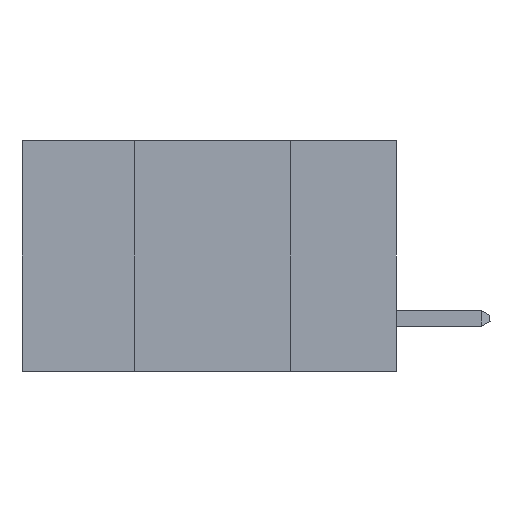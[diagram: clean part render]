
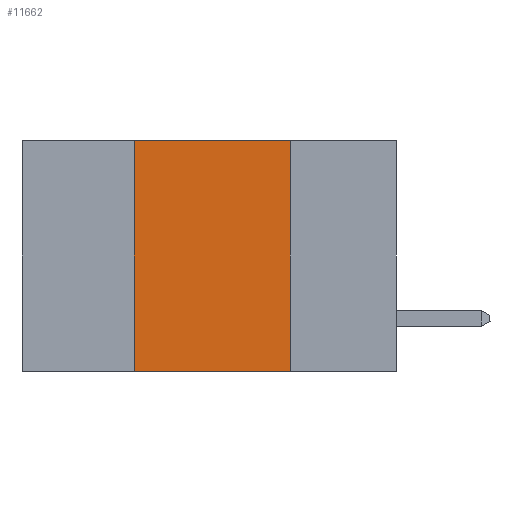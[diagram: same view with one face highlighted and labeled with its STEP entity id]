
A CAD part, left-side view. The second image highlights one B-rep face of the part: STEP entity #11662.
In plain terms, the highlighted planar face has unit normal (-1, 0, 0).
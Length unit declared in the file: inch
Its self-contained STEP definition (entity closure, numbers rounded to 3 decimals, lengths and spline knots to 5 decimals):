
#841 = VECTOR ( 'NONE', #10103, 39.37008 ) ;
#1334 = CARTESIAN_POINT ( 'NONE',  ( 0., 0.17, 0. ) ) ;
#1590 = DIRECTION ( 'NONE',  ( 0., -1., 0. ) ) ;
#1666 = EDGE_CURVE ( 'NONE', #10080, #20813, #17076, .T. ) ;
#2718 = DIRECTION ( 'NONE',  ( 0., 0., -1. ) ) ;
#3390 = VECTOR ( 'NONE', #1590, 39.37008 ) ;
#4384 = CARTESIAN_POINT ( 'NONE',  ( 0., 0.42, 0. ) ) ;
#5586 = DIRECTION ( 'NONE',  ( 0., 0., 1. ) ) ;
#5611 = EDGE_LOOP ( 'NONE', ( #13596, #7091, #16140, #17143 ) ) ;
#7091 = ORIENTED_EDGE ( 'NONE', *, *, #20095, .F. ) ;
#7186 = EDGE_CURVE ( 'NONE', #20708, #16770, #9799, .T. ) ;
#8247 = EDGE_CURVE ( 'NONE', #20708, #20813, #13792, .T. ) ;
#8627 = CARTESIAN_POINT ( 'NONE',  ( 0., 0.17, 0. ) ) ;
#9299 = VECTOR ( 'NONE', #5586, 39.37008 ) ;
#9799 = LINE ( 'NONE', #20024, #9299 ) ;
#10080 = VERTEX_POINT ( 'NONE', #8627 ) ;
#10103 = DIRECTION ( 'NONE',  ( 0., -1., 0. ) ) ;
#10778 = CARTESIAN_POINT ( 'NONE',  ( 0., 0.6, 0. ) ) ;
#11361 = CARTESIAN_POINT ( 'NONE',  ( 0., 0.6, 0. ) ) ;
#11662 = ADVANCED_FACE ( 'NONE', ( #18445 ), #20415, .F. ) ;
#12395 = DIRECTION ( 'NONE',  ( 1., 0., 0. ) ) ;
#12491 = LINE ( 'NONE', #11361, #3390 ) ;
#12782 = VECTOR ( 'NONE', #17632, 39.37008 ) ;
#12915 = CARTESIAN_POINT ( 'NONE',  ( 0., 0.42, -0.37 ) ) ;
#13135 = CARTESIAN_POINT ( 'NONE',  ( 0., 0.17, -0.37 ) ) ;
#13596 = ORIENTED_EDGE ( 'NONE', *, *, #1666, .F. ) ;
#13792 = LINE ( 'NONE', #19747, #841 ) ;
#13825 = AXIS2_PLACEMENT_3D ( 'NONE', #10778, #12395, #2718 ) ;
#16140 = ORIENTED_EDGE ( 'NONE', *, *, #7186, .F. ) ;
#16770 = VERTEX_POINT ( 'NONE', #4384 ) ;
#17076 = LINE ( 'NONE', #1334, #12782 ) ;
#17143 = ORIENTED_EDGE ( 'NONE', *, *, #8247, .T. ) ;
#17632 = DIRECTION ( 'NONE',  ( 0., 0., -1. ) ) ;
#18445 = FACE_OUTER_BOUND ( 'NONE', #5611, .T. ) ;
#19747 = CARTESIAN_POINT ( 'NONE',  ( 0., 0.6, -0.37 ) ) ;
#20024 = CARTESIAN_POINT ( 'NONE',  ( 0., 0.42, 0. ) ) ;
#20095 = EDGE_CURVE ( 'NONE', #16770, #10080, #12491, .T. ) ;
#20415 = PLANE ( 'NONE',  #13825 ) ;
#20708 = VERTEX_POINT ( 'NONE', #12915 ) ;
#20813 = VERTEX_POINT ( 'NONE', #13135 ) ;
